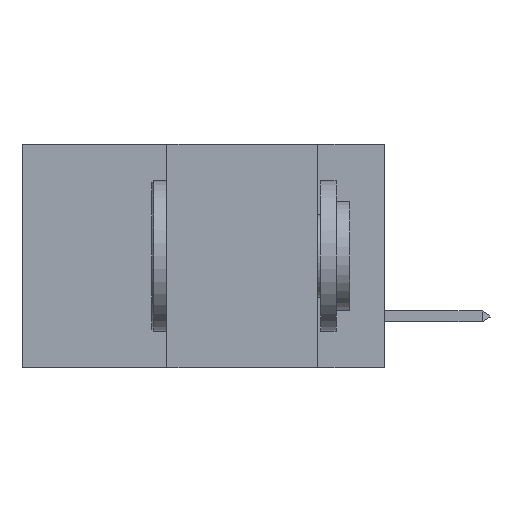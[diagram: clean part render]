
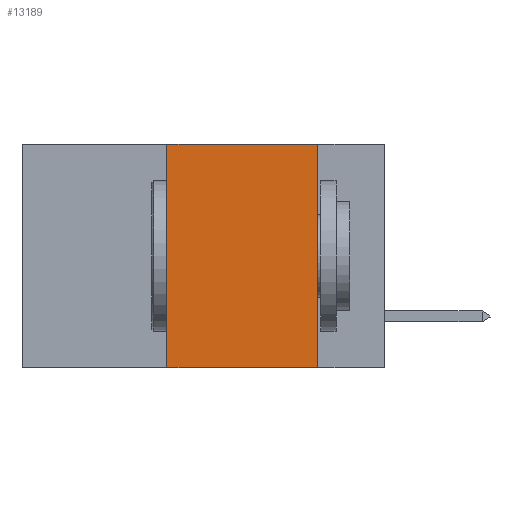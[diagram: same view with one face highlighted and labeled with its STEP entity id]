
A CAD part, left-side view. The second image highlights one B-rep face of the part: STEP entity #13189.
In plain terms, the highlighted planar face has unit normal (-1, 0, 0).
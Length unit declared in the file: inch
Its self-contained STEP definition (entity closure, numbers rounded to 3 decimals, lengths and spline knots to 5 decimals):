
#132 = VECTOR ( 'NONE', #20081, 39.37008 ) ;
#319 = DIRECTION ( 'NONE',  ( 1., 0., 0. ) ) ;
#1191 = AXIS2_PLACEMENT_3D ( 'NONE', #10057, #319, #6995 ) ;
#1762 = VECTOR ( 'NONE', #20748, 39.37008 ) ;
#3090 = EDGE_CURVE ( 'NONE', #8196, #16269, #12990, .T. ) ;
#3946 = EDGE_LOOP ( 'NONE', ( #11853, #14177, #16789, #16555 ) ) ;
#5030 = CARTESIAN_POINT ( 'NONE',  ( 0., 0.11, 0. ) ) ;
#6995 = DIRECTION ( 'NONE',  ( 0., 0., -1. ) ) ;
#7556 = CARTESIAN_POINT ( 'NONE',  ( 0., 0.6, -0.37 ) ) ;
#8196 = VERTEX_POINT ( 'NONE', #8838 ) ;
#8777 = EDGE_CURVE ( 'NONE', #19607, #16269, #17270, .T. ) ;
#8838 = CARTESIAN_POINT ( 'NONE',  ( 0., 0.11, 0. ) ) ;
#10057 = CARTESIAN_POINT ( 'NONE',  ( 0., 0.6, 0. ) ) ;
#10195 = PLANE ( 'NONE',  #1191 ) ;
#10362 = EDGE_CURVE ( 'NONE', #19586, #8196, #12282, .T. ) ;
#10617 = EDGE_CURVE ( 'NONE', #19607, #19586, #12013, .T. ) ;
#11009 = VECTOR ( 'NONE', #11321, 39.37008 ) ;
#11321 = DIRECTION ( 'NONE',  ( 0., -1., 0. ) ) ;
#11799 = CARTESIAN_POINT ( 'NONE',  ( 0., 0.36, -0.37 ) ) ;
#11853 = ORIENTED_EDGE ( 'NONE', *, *, #3090, .F. ) ;
#11934 = VECTOR ( 'NONE', #16603, 39.37008 ) ;
#12008 = CARTESIAN_POINT ( 'NONE',  ( 0., 0.36, 0. ) ) ;
#12013 = LINE ( 'NONE', #12934, #132 ) ;
#12282 = LINE ( 'NONE', #21255, #11009 ) ;
#12689 = FACE_OUTER_BOUND ( 'NONE', #3946, .T. ) ;
#12934 = CARTESIAN_POINT ( 'NONE',  ( 0., 0.36, 0. ) ) ;
#12990 = LINE ( 'NONE', #5030, #11934 ) ;
#13189 = ADVANCED_FACE ( 'NONE', ( #12689 ), #10195, .F. ) ;
#14177 = ORIENTED_EDGE ( 'NONE', *, *, #10362, .F. ) ;
#16269 = VERTEX_POINT ( 'NONE', #16615 ) ;
#16555 = ORIENTED_EDGE ( 'NONE', *, *, #8777, .T. ) ;
#16603 = DIRECTION ( 'NONE',  ( 0., 0., -1. ) ) ;
#16615 = CARTESIAN_POINT ( 'NONE',  ( 0., 0.11, -0.37 ) ) ;
#16789 = ORIENTED_EDGE ( 'NONE', *, *, #10617, .F. ) ;
#17270 = LINE ( 'NONE', #7556, #1762 ) ;
#19586 = VERTEX_POINT ( 'NONE', #12008 ) ;
#19607 = VERTEX_POINT ( 'NONE', #11799 ) ;
#20081 = DIRECTION ( 'NONE',  ( 0., 0., 1. ) ) ;
#20748 = DIRECTION ( 'NONE',  ( 0., -1., 0. ) ) ;
#21255 = CARTESIAN_POINT ( 'NONE',  ( 0., 0.6, 0. ) ) ;
